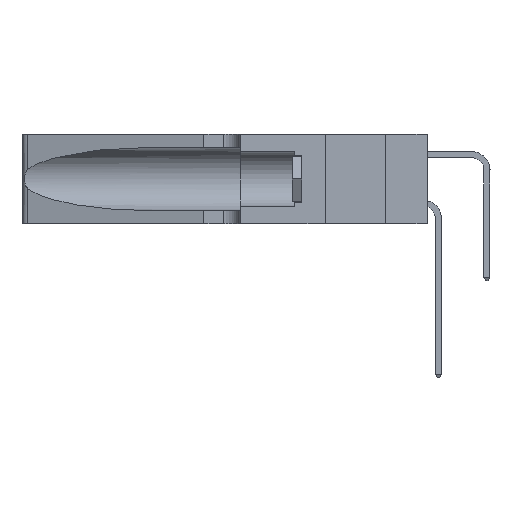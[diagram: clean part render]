
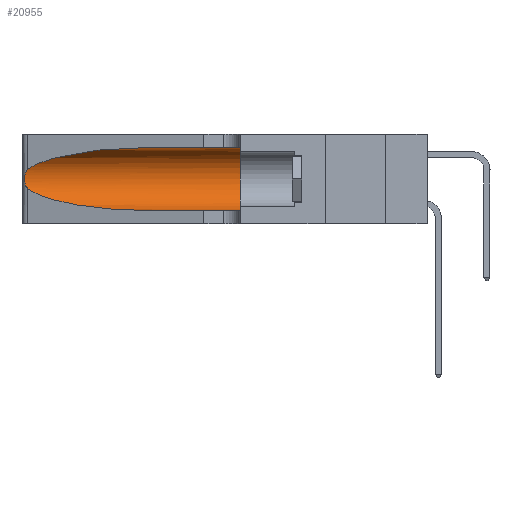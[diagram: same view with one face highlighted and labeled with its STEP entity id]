
A CAD part, left-side view. The second image highlights one B-rep face of the part: STEP entity #20955.
In plain terms, the highlighted cylindrical face has radius 3.308 mm (diameter 6.617 mm), a partial arc.
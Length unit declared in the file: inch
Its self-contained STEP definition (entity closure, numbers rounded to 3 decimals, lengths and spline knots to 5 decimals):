
#533 =( BOUNDED_CURVE ( )  B_SPLINE_CURVE ( 3, ( #21320, #24798, #20701, #31766 ),
 .UNSPECIFIED., .F., .F. ) 
 B_SPLINE_CURVE_WITH_KNOTS ( ( 4, 4 ),
 ( 3.44316, 4.71239 ),
 .UNSPECIFIED. ) 
 CURVE ( )  GEOMETRIC_REPRESENTATION_ITEM ( )  RATIONAL_B_SPLINE_CURVE ( ( 1., 0.87, 0.87, 1. ) ) 
 REPRESENTATION_ITEM ( '' )  );
#603 = CARTESIAN_POINT ( 'NONE',  ( 0.25487, 1.22718, 0.14631 ) ) ;
#762 = LINE ( 'NONE', #3302, #3997 ) ;
#918 = CARTESIAN_POINT ( 'NONE',  ( 0.26075, 1.23896, 0.178 ) ) ;
#3302 = CARTESIAN_POINT ( 'NONE',  ( 0.1305, 1.61858, 0.31525 ) ) ;
#3364 = CARTESIAN_POINT ( 'NONE',  ( 0.1305, 1.61858, 0.185 ) ) ;
#3870 = VERTEX_POINT ( 'NONE', #20736 ) ;
#3997 = VECTOR ( 'NONE', #30812, 39.37008 ) ;
#4077 = CARTESIAN_POINT ( 'NONE',  ( 0.25856, 1.23593, 0.16098 ) ) ;
#4400 = ORIENTED_EDGE ( 'NONE', *, *, #29245, .T. ) ;
#4663 = FACE_OUTER_BOUND ( 'NONE', #33768, .T. ) ;
#5098 = AXIS2_PLACEMENT_3D ( 'NONE', #28223, #39116, #31694 ) ;
#5110 = VERTEX_POINT ( 'NONE', #29682 ) ;
#6493 = CARTESIAN_POINT ( 'NONE',  ( 0.25487, 1.22718, 0.22369 ) ) ;
#7168 =( BOUNDED_CURVE ( )  B_SPLINE_CURVE ( 3, ( #41467, #31184, #31335, #41892 ),
 .UNSPECIFIED., .F., .T. ) 
 B_SPLINE_CURVE_WITH_KNOTS ( ( 4, 4 ),
 ( 1.5708, 2.84003 ),
 .UNSPECIFIED. ) 
 CURVE ( )  GEOMETRIC_REPRESENTATION_ITEM ( )  RATIONAL_B_SPLINE_CURVE ( ( 1., 0.87, 0.87, 1. ) ) 
 REPRESENTATION_ITEM ( '' )  );
#7691 = CARTESIAN_POINT ( 'NONE',  ( 0.25639, 1.23186, 0.15144 ) ) ;
#8292 = CARTESIAN_POINT ( 'NONE',  ( 0.1305, 1.61858, 0.05475 ) ) ;
#10001 = ORIENTED_EDGE ( 'NONE', *, *, #43993, .F. ) ;
#10026 = CYLINDRICAL_SURFACE ( 'NONE', #17024, 0.13025 ) ;
#11009 = CARTESIAN_POINT ( 'NONE',  ( 0.25789, 1.23486, 0.15765 ) ) ;
#12291 = ORIENTED_EDGE ( 'NONE', *, *, #12682, .T. ) ;
#12527 = EDGE_CURVE ( 'NONE', #5110, #40979, #16547, .T. ) ;
#12682 = EDGE_CURVE ( 'NONE', #3870, #38131, #21144, .T. ) ;
#15469 = ORIENTED_EDGE ( 'NONE', *, *, #12527, .T. ) ;
#16547 = B_SPLINE_CURVE_WITH_KNOTS ( 'NONE', 3,
 ( #6493, #37618, #38852, #21605, #38701, #17945, #38382, #918, #39001, #4077, #11009, #7691, #18243, #603 ),
 .UNSPECIFIED., .F., .F.,
 ( 4, 2, 2, 2, 2, 2, 4 ),
 ( 0., 0.00027, 0.00053, 0.00107, 0.0016, 0.00187, 0.00214 ),
 .UNSPECIFIED. ) ;
#17024 = AXIS2_PLACEMENT_3D ( 'NONE', #3364, #23880, #30870 ) ;
#17945 = CARTESIAN_POINT ( 'NONE',  ( 0.26018, 1.23835, 0.19895 ) ) ;
#18243 = CARTESIAN_POINT ( 'NONE',  ( 0.25555, 1.22993, 0.14849 ) ) ;
#20701 = CARTESIAN_POINT ( 'NONE',  ( 0.18966, 0.96281, 0.05475 ) ) ;
#20736 = CARTESIAN_POINT ( 'NONE',  ( 0.1305, 0.72297, 0.05475 ) ) ;
#20817 = CARTESIAN_POINT ( 'NONE',  ( 0.1305, 0.35, 0.31525 ) ) ;
#20955 = ADVANCED_FACE ( 'NONE', ( #4663 ), #10026, .F. ) ;
#21144 = LINE ( 'NONE', #8292, #39542 ) ;
#21320 = CARTESIAN_POINT ( 'NONE',  ( 0.25487, 1.22718, 0.14631 ) ) ;
#21605 = CARTESIAN_POINT ( 'NONE',  ( 0.25787, 1.23484, 0.2124 ) ) ;
#22591 = ORIENTED_EDGE ( 'NONE', *, *, #34125, .T. ) ;
#23880 = DIRECTION ( 'NONE',  ( 0., -1., 0. ) ) ;
#24538 = VERTEX_POINT ( 'NONE', #20817 ) ;
#24798 = CARTESIAN_POINT ( 'NONE',  ( 0.2373, 1.15595, 0.08982 ) ) ;
#26191 = CARTESIAN_POINT ( 'NONE',  ( 0.25487, 1.22718, 0.14631 ) ) ;
#28223 = CARTESIAN_POINT ( 'NONE',  ( 0.1305, 0.35, 0.185 ) ) ;
#28367 = CARTESIAN_POINT ( 'NONE',  ( 0.1305, 0.35, 0.05475 ) ) ;
#29245 = EDGE_CURVE ( 'NONE', #40979, #3870, #533, .T. ) ;
#29682 = CARTESIAN_POINT ( 'NONE',  ( 0.25487, 1.22718, 0.22369 ) ) ;
#30812 = DIRECTION ( 'NONE',  ( 0., -1., 0. ) ) ;
#30870 = DIRECTION ( 'NONE',  ( 0., 0., -1. ) ) ;
#31184 = CARTESIAN_POINT ( 'NONE',  ( 0.18966, 0.96281, 0.31525 ) ) ;
#31335 = CARTESIAN_POINT ( 'NONE',  ( 0.2373, 1.15595, 0.28018 ) ) ;
#31694 = DIRECTION ( 'NONE',  ( 0., 0., 1. ) ) ;
#31766 = CARTESIAN_POINT ( 'NONE',  ( 0.1305, 0.72297, 0.05475 ) ) ;
#31860 = CARTESIAN_POINT ( 'NONE',  ( 0.1305, 0.72297, 0.31525 ) ) ;
#33768 = EDGE_LOOP ( 'NONE', ( #22591, #15469, #4400, #12291, #10001, #40497 ) ) ;
#34125 = EDGE_CURVE ( 'NONE', #35337, #5110, #7168, .T. ) ;
#35337 = VERTEX_POINT ( 'NONE', #31860 ) ;
#35806 = DIRECTION ( 'NONE',  ( 0., -1., 0. ) ) ;
#37149 = CIRCLE ( 'NONE', #5098, 0.13025 ) ;
#37618 = CARTESIAN_POINT ( 'NONE',  ( 0.25555, 1.22994, 0.2215 ) ) ;
#38131 = VERTEX_POINT ( 'NONE', #28367 ) ;
#38382 = CARTESIAN_POINT ( 'NONE',  ( 0.26075, 1.23896, 0.19203 ) ) ;
#38701 = CARTESIAN_POINT ( 'NONE',  ( 0.25854, 1.2359, 0.20912 ) ) ;
#38852 = CARTESIAN_POINT ( 'NONE',  ( 0.25639, 1.23184, 0.21858 ) ) ;
#39001 = CARTESIAN_POINT ( 'NONE',  ( 0.26017, 1.23833, 0.17102 ) ) ;
#39116 = DIRECTION ( 'NONE',  ( 0., 1., 0. ) ) ;
#39542 = VECTOR ( 'NONE', #35806, 39.37008 ) ;
#39800 = EDGE_CURVE ( 'NONE', #35337, #24538, #762, .T. ) ;
#40497 = ORIENTED_EDGE ( 'NONE', *, *, #39800, .F. ) ;
#40979 = VERTEX_POINT ( 'NONE', #26191 ) ;
#41467 = CARTESIAN_POINT ( 'NONE',  ( 0.1305, 0.72297, 0.31525 ) ) ;
#41892 = CARTESIAN_POINT ( 'NONE',  ( 0.25487, 1.22718, 0.22369 ) ) ;
#43993 = EDGE_CURVE ( 'NONE', #24538, #38131, #37149, .T. ) ;
